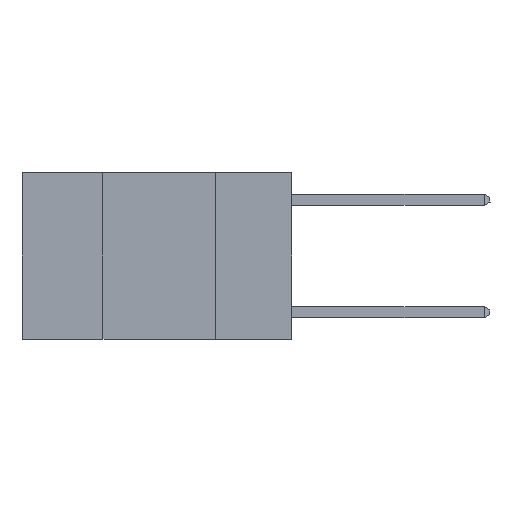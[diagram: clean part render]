
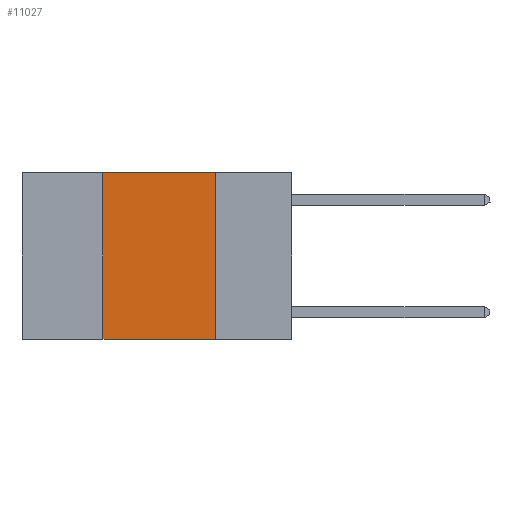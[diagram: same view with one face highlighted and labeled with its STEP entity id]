
A CAD part, left-side view. The second image highlights one B-rep face of the part: STEP entity #11027.
In plain terms, the highlighted planar face has unit normal (-1, 0, 0).
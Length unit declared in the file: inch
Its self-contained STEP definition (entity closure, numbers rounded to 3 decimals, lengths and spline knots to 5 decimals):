
#3 = VECTOR ( 'NONE', #12503, 39.37008 ) ;
#244 = CARTESIAN_POINT ( 'NONE',  ( 0., 0.42, 0. ) ) ;
#487 = EDGE_CURVE ( 'NONE', #12492, #3360, #6144, .T. ) ;
#550 = EDGE_CURVE ( 'NONE', #9971, #12245, #5416, .T. ) ;
#1479 = ORIENTED_EDGE ( 'NONE', *, *, #487, .F. ) ;
#1650 = CARTESIAN_POINT ( 'NONE',  ( 0., 0.42, 0. ) ) ;
#1679 = EDGE_CURVE ( 'NONE', #3360, #12245, #9896, .T. ) ;
#3027 = VECTOR ( 'NONE', #7613, 39.37008 ) ;
#3360 = VERTEX_POINT ( 'NONE', #3942 ) ;
#3942 = CARTESIAN_POINT ( 'NONE',  ( 0., 0.17, 0. ) ) ;
#4006 = ORIENTED_EDGE ( 'NONE', *, *, #1679, .F. ) ;
#4027 = DIRECTION ( 'NONE',  ( 1., 0., 0. ) ) ;
#4827 = FACE_OUTER_BOUND ( 'NONE', #11555, .T. ) ;
#5416 = LINE ( 'NONE', #6428, #13033 ) ;
#6144 = LINE ( 'NONE', #12612, #3 ) ;
#6428 = CARTESIAN_POINT ( 'NONE',  ( 0., 0.6, -0.37 ) ) ;
#6702 = VECTOR ( 'NONE', #9138, 39.37008 ) ;
#7597 = CARTESIAN_POINT ( 'NONE',  ( 0., 0.6, 0. ) ) ;
#7613 = DIRECTION ( 'NONE',  ( 0., 0., 1. ) ) ;
#8329 = ORIENTED_EDGE ( 'NONE', *, *, #12421, .F. ) ;
#9138 = DIRECTION ( 'NONE',  ( 0., 0., -1. ) ) ;
#9371 = DIRECTION ( 'NONE',  ( 0., -1., 0. ) ) ;
#9896 = LINE ( 'NONE', #15271, #6702 ) ;
#9971 = VERTEX_POINT ( 'NONE', #15219 ) ;
#11027 = ADVANCED_FACE ( 'NONE', ( #4827 ), #11260, .F. ) ;
#11260 = PLANE ( 'NONE',  #13178 ) ;
#11555 = EDGE_LOOP ( 'NONE', ( #4006, #1479, #8329, #12964 ) ) ;
#12245 = VERTEX_POINT ( 'NONE', #12666 ) ;
#12421 = EDGE_CURVE ( 'NONE', #9971, #12492, #13132, .T. ) ;
#12492 = VERTEX_POINT ( 'NONE', #1650 ) ;
#12503 = DIRECTION ( 'NONE',  ( 0., -1., 0. ) ) ;
#12509 = DIRECTION ( 'NONE',  ( 0., 0., -1. ) ) ;
#12612 = CARTESIAN_POINT ( 'NONE',  ( 0., 0.6, 0. ) ) ;
#12666 = CARTESIAN_POINT ( 'NONE',  ( 0., 0.17, -0.37 ) ) ;
#12964 = ORIENTED_EDGE ( 'NONE', *, *, #550, .T. ) ;
#13033 = VECTOR ( 'NONE', #9371, 39.37008 ) ;
#13132 = LINE ( 'NONE', #244, #3027 ) ;
#13178 = AXIS2_PLACEMENT_3D ( 'NONE', #7597, #4027, #12509 ) ;
#15219 = CARTESIAN_POINT ( 'NONE',  ( 0., 0.42, -0.37 ) ) ;
#15271 = CARTESIAN_POINT ( 'NONE',  ( 0., 0.17, 0. ) ) ;
